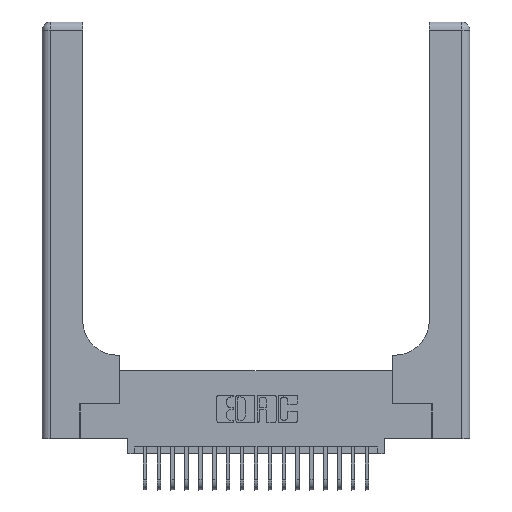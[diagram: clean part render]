
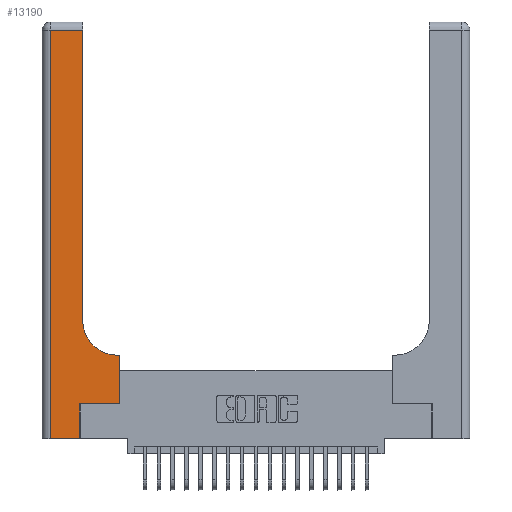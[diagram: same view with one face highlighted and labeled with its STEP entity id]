
A CAD part, top view. The second image highlights one B-rep face of the part: STEP entity #13190.
In plain terms, the highlighted planar face has unit normal (0, 0, 1).
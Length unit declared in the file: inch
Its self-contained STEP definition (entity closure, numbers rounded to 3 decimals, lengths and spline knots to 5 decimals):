
#225 = VERTEX_POINT ( 'NONE', #19033 ) ;
#282 = DIRECTION ( 'NONE',  ( 0., -1., 0. ) ) ;
#371 = EDGE_CURVE ( 'NONE', #5413, #1650, #1839, .T. ) ;
#564 = VECTOR ( 'NONE', #13871, 39.37008 ) ;
#726 = VECTOR ( 'NONE', #1103, 39.37008 ) ;
#731 = ORIENTED_EDGE ( 'NONE', *, *, #10275, .T. ) ;
#1103 = DIRECTION ( 'NONE',  ( -1., 0., 0. ) ) ;
#1132 = VERTEX_POINT ( 'NONE', #1780 ) ;
#1513 = CARTESIAN_POINT ( 'NONE',  ( 0.5415, 0.85, 0.37 ) ) ;
#1650 = VERTEX_POINT ( 'NONE', #20858 ) ;
#1780 = CARTESIAN_POINT ( 'NONE',  ( 0.269, 0., 0.37 ) ) ;
#1839 = LINE ( 'NONE', #21042, #10189 ) ;
#2327 = LINE ( 'NONE', #18688, #7264 ) ;
#2825 = PLANE ( 'NONE',  #8470 ) ;
#3175 = AXIS2_PLACEMENT_3D ( 'NONE', #1513, #13182, #3188 ) ;
#3188 = DIRECTION ( 'NONE',  ( 1., 0., 0. ) ) ;
#3583 = LINE ( 'NONE', #13316, #8015 ) ;
#3746 = CIRCLE ( 'NONE', #3175, 0.25 ) ;
#3969 = CARTESIAN_POINT ( 'NONE',  ( 0.2915, 3., 0.37 ) ) ;
#4129 = LINE ( 'NONE', #5325, #21317 ) ;
#4482 = DIRECTION ( 'NONE',  ( -1., 0., 0. ) ) ;
#4594 = LINE ( 'NONE', #11079, #726 ) ;
#5008 = EDGE_CURVE ( 'NONE', #9424, #16633, #3746, .T. ) ;
#5325 = CARTESIAN_POINT ( 'NONE',  ( 0.269, 0., 0.37 ) ) ;
#5413 = VERTEX_POINT ( 'NONE', #19869 ) ;
#5590 = VECTOR ( 'NONE', #282, 39.37008 ) ;
#6090 = CARTESIAN_POINT ( 'NONE',  ( 0., 3., 0.37 ) ) ;
#6918 = DIRECTION ( 'NONE',  ( -1., 0., 0. ) ) ;
#7148 = ORIENTED_EDGE ( 'NONE', *, *, #371, .T. ) ;
#7197 = CARTESIAN_POINT ( 'NONE',  ( 0.5585, 0.25, 0.37 ) ) ;
#7250 = CARTESIAN_POINT ( 'NONE',  ( 0.2915, 0.85, 0.37 ) ) ;
#7264 = VECTOR ( 'NONE', #6918, 39.37008 ) ;
#7472 = VECTOR ( 'NONE', #12383, 39.37008 ) ;
#7985 = LINE ( 'NONE', #3969, #7472 ) ;
#8015 = VECTOR ( 'NONE', #18337, 39.37008 ) ;
#8470 = AXIS2_PLACEMENT_3D ( 'NONE', #6090, #14508, #4482 ) ;
#8717 = DIRECTION ( 'NONE',  ( 0., 1., 0. ) ) ;
#8788 = CARTESIAN_POINT ( 'NONE',  ( 0.5415, 0.6, 0.37 ) ) ;
#8900 = LINE ( 'NONE', #7197, #564 ) ;
#8918 = ORIENTED_EDGE ( 'NONE', *, *, #19352, .T. ) ;
#9424 = VERTEX_POINT ( 'NONE', #8788 ) ;
#9512 = ORIENTED_EDGE ( 'NONE', *, *, #16196, .T. ) ;
#9608 = CARTESIAN_POINT ( 'NONE',  ( 0.2915, 2.94, 0.37 ) ) ;
#10141 = ORIENTED_EDGE ( 'NONE', *, *, #5008, .T. ) ;
#10189 = VECTOR ( 'NONE', #19384, 39.37008 ) ;
#10275 = EDGE_CURVE ( 'NONE', #18636, #225, #4594, .T. ) ;
#10592 = VERTEX_POINT ( 'NONE', #16807 ) ;
#10660 = ORIENTED_EDGE ( 'NONE', *, *, #11576, .T. ) ;
#11079 = CARTESIAN_POINT ( 'NONE',  ( 0., 2.94, 0.37 ) ) ;
#11576 = EDGE_CURVE ( 'NONE', #225, #10592, #14497, .T. ) ;
#12383 = DIRECTION ( 'NONE',  ( 0., 1., 0. ) ) ;
#12672 = CARTESIAN_POINT ( 'NONE',  ( 0.5585, 0.6, 0.37 ) ) ;
#13182 = DIRECTION ( 'NONE',  ( 0., 0., -1. ) ) ;
#13190 = ADVANCED_FACE ( 'NONE', ( #14485 ), #2825, .F. ) ;
#13316 = CARTESIAN_POINT ( 'NONE',  ( 0., 0., 0.37 ) ) ;
#13871 = DIRECTION ( 'NONE',  ( 0., 1., 0. ) ) ;
#14485 = FACE_OUTER_BOUND ( 'NONE', #16421, .T. ) ;
#14497 = LINE ( 'NONE', #15217, #5590 ) ;
#14508 = DIRECTION ( 'NONE',  ( 0., 0., -1. ) ) ;
#15217 = CARTESIAN_POINT ( 'NONE',  ( 0.06, 3., 0.37 ) ) ;
#16196 = EDGE_CURVE ( 'NONE', #1650, #21324, #8900, .T. ) ;
#16421 = EDGE_LOOP ( 'NONE', ( #8918, #731, #10660, #20980, #18004, #7148, #9512, #18308, #10141 ) ) ;
#16633 = VERTEX_POINT ( 'NONE', #7250 ) ;
#16807 = CARTESIAN_POINT ( 'NONE',  ( 0.06, 0., 0.37 ) ) ;
#17185 = EDGE_CURVE ( 'NONE', #21324, #9424, #2327, .T. ) ;
#18004 = ORIENTED_EDGE ( 'NONE', *, *, #18392, .T. ) ;
#18308 = ORIENTED_EDGE ( 'NONE', *, *, #17185, .T. ) ;
#18337 = DIRECTION ( 'NONE',  ( 1., 0., 0. ) ) ;
#18392 = EDGE_CURVE ( 'NONE', #1132, #5413, #4129, .T. ) ;
#18636 = VERTEX_POINT ( 'NONE', #9608 ) ;
#18688 = CARTESIAN_POINT ( 'NONE',  ( 0.2915, 0.6, 0.37 ) ) ;
#19033 = CARTESIAN_POINT ( 'NONE',  ( 0.06, 2.94, 0.37 ) ) ;
#19352 = EDGE_CURVE ( 'NONE', #16633, #18636, #7985, .T. ) ;
#19384 = DIRECTION ( 'NONE',  ( 1., 0., 0. ) ) ;
#19588 = EDGE_CURVE ( 'NONE', #10592, #1132, #3583, .T. ) ;
#19869 = CARTESIAN_POINT ( 'NONE',  ( 0.269, 0.25, 0.37 ) ) ;
#20858 = CARTESIAN_POINT ( 'NONE',  ( 0.5585, 0.25, 0.37 ) ) ;
#20980 = ORIENTED_EDGE ( 'NONE', *, *, #19588, .T. ) ;
#21042 = CARTESIAN_POINT ( 'NONE',  ( 0.269, 0.25, 0.37 ) ) ;
#21317 = VECTOR ( 'NONE', #8717, 39.37008 ) ;
#21324 = VERTEX_POINT ( 'NONE', #12672 ) ;
